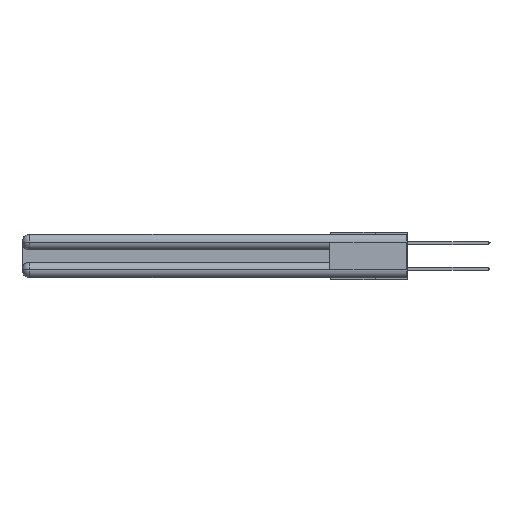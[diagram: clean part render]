
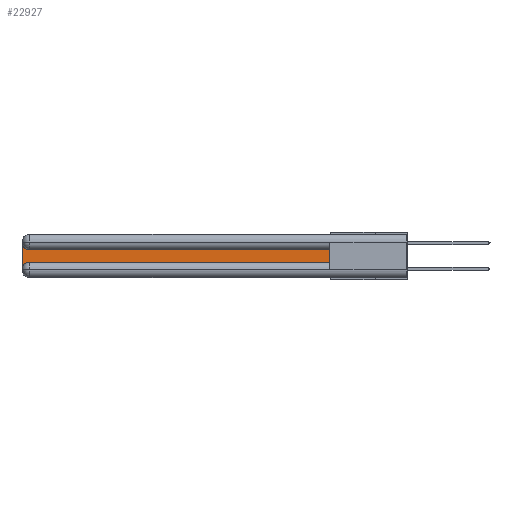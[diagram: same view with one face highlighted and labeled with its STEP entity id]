
A CAD part, left-side view. The second image highlights one B-rep face of the part: STEP entity #22927.
In plain terms, the highlighted planar face has unit normal (-1, 0, 0).
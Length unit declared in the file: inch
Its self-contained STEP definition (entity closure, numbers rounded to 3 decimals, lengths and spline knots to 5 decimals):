
#452 = VERTEX_POINT ( 'NONE', #3625 ) ;
#2923 = LINE ( 'NONE', #2957, #6461 ) ;
#2957 = CARTESIAN_POINT ( 'NONE',  ( 0.075, 3., -0.2175 ) ) ;
#3625 = CARTESIAN_POINT ( 'NONE',  ( 0.075, 2.94, -0.1225 ) ) ;
#3997 = DIRECTION ( 'NONE',  ( 0., 1., 0. ) ) ;
#4468 = VECTOR ( 'NONE', #3997, 39.37008 ) ;
#5302 = DIRECTION ( 'NONE',  ( 0., -1., 0. ) ) ;
#5881 = EDGE_CURVE ( 'NONE', #452, #11150, #22869, .T. ) ;
#6315 = AXIS2_PLACEMENT_3D ( 'NONE', #9547, #31799, #31915 ) ;
#6461 = VECTOR ( 'NONE', #23431, 39.37008 ) ;
#7247 = CARTESIAN_POINT ( 'NONE',  ( 0.075, 2.94, -0.2775 ) ) ;
#7690 = VERTEX_POINT ( 'NONE', #9869 ) ;
#9547 = CARTESIAN_POINT ( 'NONE',  ( 0.075, 2.94, -0.0625 ) ) ;
#9578 = CARTESIAN_POINT ( 'NONE',  ( 0.075, 0.6, -0.2175 ) ) ;
#9869 = CARTESIAN_POINT ( 'NONE',  ( 0.075, 2.94, -0.2175 ) ) ;
#10069 = DIRECTION ( 'NONE',  ( 0., 0., -1. ) ) ;
#10117 = EDGE_CURVE ( 'NONE', #20974, #452, #29751, .T. ) ;
#10772 = ORIENTED_EDGE ( 'NONE', *, *, #11435, .T. ) ;
#11150 = VERTEX_POINT ( 'NONE', #24543 ) ;
#11412 = FACE_OUTER_BOUND ( 'NONE', #21221, .T. ) ;
#11435 = EDGE_CURVE ( 'NONE', #11150, #25073, #2923, .T. ) ;
#12065 = VERTEX_POINT ( 'NONE', #9578 ) ;
#12672 = EDGE_CURVE ( 'NONE', #7690, #12065, #16089, .T. ) ;
#12703 = CARTESIAN_POINT ( 'NONE',  ( 0.075, 3., -0.1225 ) ) ;
#13109 = AXIS2_PLACEMENT_3D ( 'NONE', #7247, #22103, #20105 ) ;
#15150 = CIRCLE ( 'NONE', #13109, 0.06 ) ;
#16089 = LINE ( 'NONE', #18262, #30336 ) ;
#16620 = DIRECTION ( 'NONE',  ( 0., 0., 1. ) ) ;
#16746 = ORIENTED_EDGE ( 'NONE', *, *, #20238, .T. ) ;
#18262 = CARTESIAN_POINT ( 'NONE',  ( 0.075, 0.6, -0.2175 ) ) ;
#19650 = ORIENTED_EDGE ( 'NONE', *, *, #12672, .T. ) ;
#20105 = DIRECTION ( 'NONE',  ( 0., 0., -1. ) ) ;
#20238 = EDGE_CURVE ( 'NONE', #25073, #7690, #15150, .T. ) ;
#20974 = VERTEX_POINT ( 'NONE', #24977 ) ;
#21221 = EDGE_LOOP ( 'NONE', ( #23527, #21817, #10772, #16746, #19650, #32610 ) ) ;
#21432 = CARTESIAN_POINT ( 'NONE',  ( 0.075, 0.6, -0.2175 ) ) ;
#21817 = ORIENTED_EDGE ( 'NONE', *, *, #5881, .T. ) ;
#22103 = DIRECTION ( 'NONE',  ( 1., 0., 0. ) ) ;
#22869 = CIRCLE ( 'NONE', #6315, 0.06 ) ;
#22927 = ADVANCED_FACE ( 'NONE', ( #11412 ), #32338, .F. ) ;
#23431 = DIRECTION ( 'NONE',  ( 0., 0., -1. ) ) ;
#23527 = ORIENTED_EDGE ( 'NONE', *, *, #10117, .T. ) ;
#24041 = EDGE_CURVE ( 'NONE', #12065, #20974, #25930, .T. ) ;
#24543 = CARTESIAN_POINT ( 'NONE',  ( 0.075, 3., -0.0625 ) ) ;
#24605 = CARTESIAN_POINT ( 'NONE',  ( 0.075, 3., -0.2775 ) ) ;
#24977 = CARTESIAN_POINT ( 'NONE',  ( 0.075, 0.6, -0.1225 ) ) ;
#25073 = VERTEX_POINT ( 'NONE', #24605 ) ;
#25930 = LINE ( 'NONE', #21432, #28695 ) ;
#28695 = VECTOR ( 'NONE', #16620, 39.37008 ) ;
#29751 = LINE ( 'NONE', #31660, #4468 ) ;
#29933 = DIRECTION ( 'NONE',  ( 1., 0., 0. ) ) ;
#30336 = VECTOR ( 'NONE', #5302, 39.37008 ) ;
#31660 = CARTESIAN_POINT ( 'NONE',  ( 0.075, 0.6, -0.1225 ) ) ;
#31799 = DIRECTION ( 'NONE',  ( 1., 0., 0. ) ) ;
#31915 = DIRECTION ( 'NONE',  ( 0., 0., -1. ) ) ;
#32338 = PLANE ( 'NONE',  #32377 ) ;
#32377 = AXIS2_PLACEMENT_3D ( 'NONE', #12703, #29933, #10069 ) ;
#32610 = ORIENTED_EDGE ( 'NONE', *, *, #24041, .T. ) ;
